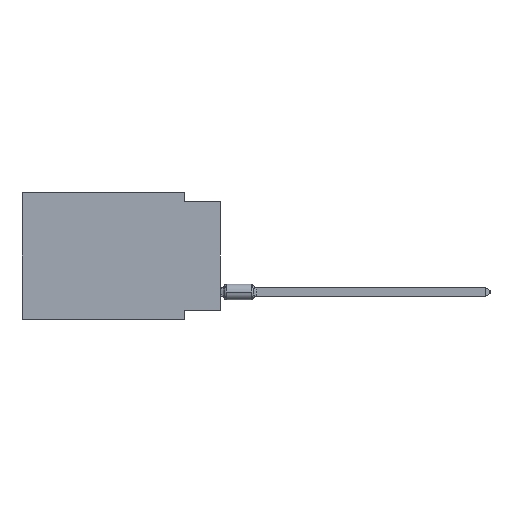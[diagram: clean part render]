
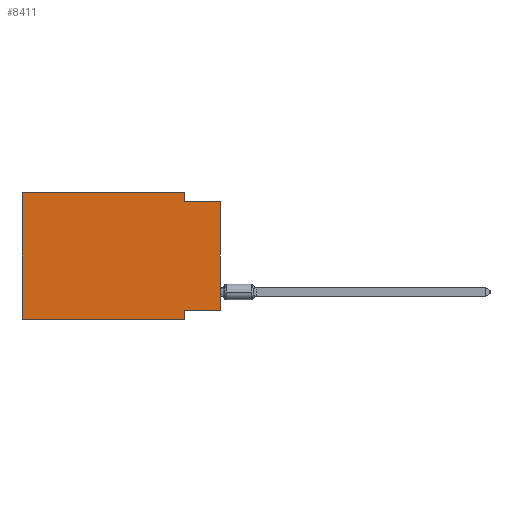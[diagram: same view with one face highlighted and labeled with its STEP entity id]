
A CAD part, left-side view. The second image highlights one B-rep face of the part: STEP entity #8411.
In plain terms, the highlighted planar face has unit normal (-1, 0, 0).
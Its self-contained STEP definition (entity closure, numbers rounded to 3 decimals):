
#6 = CARTESIAN_POINT ( 'NONE',  ( 0., 13.97, 0. ) ) ;
#192 = CARTESIAN_POINT ( 'NONE',  ( 0., 13.97, -8.89 ) ) ;
#296 = VERTEX_POINT ( 'NONE', #6143 ) ;
#650 = VECTOR ( 'NONE', #3466, 1000. ) ;
#701 = CARTESIAN_POINT ( 'NONE',  ( 0., 13.97, -8.89 ) ) ;
#903 = CARTESIAN_POINT ( 'NONE',  ( 0., 0., -0.635 ) ) ;
#984 = ORIENTED_EDGE ( 'NONE', *, *, #9116, .T. ) ;
#995 = VERTEX_POINT ( 'NONE', #5652 ) ;
#1135 = DIRECTION ( 'NONE',  ( 0., 0., -1. ) ) ;
#1255 = CARTESIAN_POINT ( 'NONE',  ( 0., 2.54, 0. ) ) ;
#1262 = VECTOR ( 'NONE', #8115, 1000. ) ;
#2317 = EDGE_LOOP ( 'NONE', ( #984, #4935, #12606, #4598, #9779, #2832, #11370, #3639 ) ) ;
#2400 = VECTOR ( 'NONE', #5125, 1000. ) ;
#2442 = EDGE_CURVE ( 'NONE', #7094, #11392, #11618, .T. ) ;
#2555 = CARTESIAN_POINT ( 'NONE',  ( 0., 2.54, -8.255 ) ) ;
#2832 = ORIENTED_EDGE ( 'NONE', *, *, #10061, .T. ) ;
#3342 = DIRECTION ( 'NONE',  ( 0., 0., 1. ) ) ;
#3466 = DIRECTION ( 'NONE',  ( 0., 0., -1. ) ) ;
#3516 = DIRECTION ( 'NONE',  ( 1., 0., 0. ) ) ;
#3639 = ORIENTED_EDGE ( 'NONE', *, *, #11935, .F. ) ;
#4019 = CARTESIAN_POINT ( 'NONE',  ( 0., 0., -8.255 ) ) ;
#4216 = CARTESIAN_POINT ( 'NONE',  ( 0., 0., 0. ) ) ;
#4278 = EDGE_CURVE ( 'NONE', #995, #8191, #8730, .T. ) ;
#4598 = ORIENTED_EDGE ( 'NONE', *, *, #4278, .F. ) ;
#4858 = CARTESIAN_POINT ( 'NONE',  ( 0., 2.54, -8.89 ) ) ;
#4924 = VECTOR ( 'NONE', #12846, 1000. ) ;
#4935 = ORIENTED_EDGE ( 'NONE', *, *, #6329, .F. ) ;
#5052 = VECTOR ( 'NONE', #5178, 1000. ) ;
#5125 = DIRECTION ( 'NONE',  ( 0., 0., 1. ) ) ;
#5178 = DIRECTION ( 'NONE',  ( 0., 1., 0. ) ) ;
#5184 = LINE ( 'NONE', #4216, #5240 ) ;
#5240 = VECTOR ( 'NONE', #3342, 1000. ) ;
#5248 = LINE ( 'NONE', #7229, #1262 ) ;
#5599 = VERTEX_POINT ( 'NONE', #192 ) ;
#5652 = CARTESIAN_POINT ( 'NONE',  ( 0., 13.97, 0. ) ) ;
#6143 = CARTESIAN_POINT ( 'NONE',  ( 0., 2.54, -0.635 ) ) ;
#6329 = EDGE_CURVE ( 'NONE', #296, #10172, #5248, .T. ) ;
#6449 = LINE ( 'NONE', #10549, #650 ) ;
#6710 = FACE_OUTER_BOUND ( 'NONE', #2317, .T. ) ;
#7094 = VERTEX_POINT ( 'NONE', #2555 ) ;
#7229 = CARTESIAN_POINT ( 'NONE',  ( 0., 0., -0.635 ) ) ;
#7708 = CARTESIAN_POINT ( 'NONE',  ( 0., 13.97, 0. ) ) ;
#7793 = CARTESIAN_POINT ( 'NONE',  ( 0., 13.97, 0. ) ) ;
#7822 = EDGE_CURVE ( 'NONE', #8191, #296, #6449, .T. ) ;
#8115 = DIRECTION ( 'NONE',  ( 0., -1., 0. ) ) ;
#8191 = VERTEX_POINT ( 'NONE', #1255 ) ;
#8411 = ADVANCED_FACE ( 'NONE', ( #6710 ), #9021, .F. ) ;
#8459 = CARTESIAN_POINT ( 'NONE',  ( 0., 0., -8.255 ) ) ;
#8730 = LINE ( 'NONE', #7708, #4924 ) ;
#9008 = DIRECTION ( 'NONE',  ( 0., -1., 0. ) ) ;
#9021 = PLANE ( 'NONE',  #9791 ) ;
#9116 = EDGE_CURVE ( 'NONE', #12635, #10172, #5184, .T. ) ;
#9355 = VECTOR ( 'NONE', #9008, 1000. ) ;
#9388 = CARTESIAN_POINT ( 'NONE',  ( 0., 2.54, -8.89 ) ) ;
#9779 = ORIENTED_EDGE ( 'NONE', *, *, #10112, .F. ) ;
#9791 = AXIS2_PLACEMENT_3D ( 'NONE', #7793, #3516, #10811 ) ;
#10034 = LINE ( 'NONE', #701, #9355 ) ;
#10061 = EDGE_CURVE ( 'NONE', #5599, #11392, #10034, .T. ) ;
#10112 = EDGE_CURVE ( 'NONE', #5599, #995, #12308, .T. ) ;
#10172 = VERTEX_POINT ( 'NONE', #903 ) ;
#10549 = CARTESIAN_POINT ( 'NONE',  ( 0., 2.54, 0. ) ) ;
#10811 = DIRECTION ( 'NONE',  ( 0., 0., -1. ) ) ;
#11370 = ORIENTED_EDGE ( 'NONE', *, *, #2442, .F. ) ;
#11392 = VERTEX_POINT ( 'NONE', #4858 ) ;
#11406 = VECTOR ( 'NONE', #1135, 1000. ) ;
#11618 = LINE ( 'NONE', #9388, #11406 ) ;
#11935 = EDGE_CURVE ( 'NONE', #12635, #7094, #12487, .T. ) ;
#12308 = LINE ( 'NONE', #6, #2400 ) ;
#12487 = LINE ( 'NONE', #4019, #5052 ) ;
#12606 = ORIENTED_EDGE ( 'NONE', *, *, #7822, .F. ) ;
#12635 = VERTEX_POINT ( 'NONE', #8459 ) ;
#12846 = DIRECTION ( 'NONE',  ( 0., -1., 0. ) ) ;
